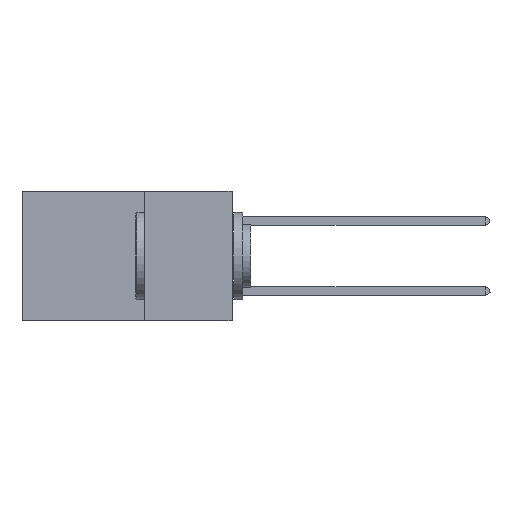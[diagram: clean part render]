
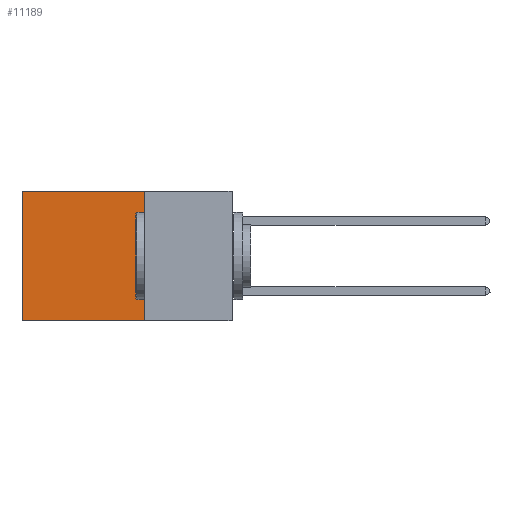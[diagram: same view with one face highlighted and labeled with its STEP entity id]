
A CAD part, left-side view. The second image highlights one B-rep face of the part: STEP entity #11189.
In plain terms, the highlighted planar face has unit normal (-1, 0, 0).
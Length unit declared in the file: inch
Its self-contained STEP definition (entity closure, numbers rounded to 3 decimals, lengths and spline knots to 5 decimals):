
#3844 = VECTOR ( 'NONE', #5964, 39.37008 ) ;
#5964 = DIRECTION ( 'NONE',  ( 0., 0., -1. ) ) ;
#8253 = EDGE_CURVE ( 'NONE', #15216, #16687, #18458, .T. ) ;
#8690 = CARTESIAN_POINT ( 'NONE',  ( 0.2875, 0.25, 0. ) ) ;
#9561 = EDGE_LOOP ( 'NONE', ( #16670, #21489, #13626, #18859 ) ) ;
#10514 = CARTESIAN_POINT ( 'NONE',  ( 0.2875, 0.25, 0. ) ) ;
#10618 = EDGE_CURVE ( 'NONE', #20994, #16687, #25148, .T. ) ;
#11189 = ADVANCED_FACE ( 'NONE', ( #21681 ), #18663, .F. ) ;
#11270 = VECTOR ( 'NONE', #27126, 39.37008 ) ;
#11901 = CARTESIAN_POINT ( 'NONE',  ( 0.2875, 0.25, 0. ) ) ;
#11990 = CARTESIAN_POINT ( 'NONE',  ( 0.2875, 0.25, -0.37 ) ) ;
#13626 = ORIENTED_EDGE ( 'NONE', *, *, #20654, .F. ) ;
#14032 = CARTESIAN_POINT ( 'NONE',  ( 0.2875, 0.6, 0. ) ) ;
#14743 = LINE ( 'NONE', #25379, #3844 ) ;
#15216 = VERTEX_POINT ( 'NONE', #17450 ) ;
#16177 = DIRECTION ( 'NONE',  ( 1., 0., 0. ) ) ;
#16329 = CARTESIAN_POINT ( 'NONE',  ( 0.2875, 0.6, -0.37 ) ) ;
#16400 = CARTESIAN_POINT ( 'NONE',  ( 0.2875, 0.6, 0. ) ) ;
#16670 = ORIENTED_EDGE ( 'NONE', *, *, #10618, .T. ) ;
#16687 = VERTEX_POINT ( 'NONE', #16329 ) ;
#17450 = CARTESIAN_POINT ( 'NONE',  ( 0.2875, 0.25, -0.37 ) ) ;
#18383 = AXIS2_PLACEMENT_3D ( 'NONE', #11901, #16177, #22835 ) ;
#18458 = LINE ( 'NONE', #11990, #11270 ) ;
#18600 = DIRECTION ( 'NONE',  ( 0., 0., -1. ) ) ;
#18604 = VERTEX_POINT ( 'NONE', #10514 ) ;
#18663 = PLANE ( 'NONE',  #18383 ) ;
#18859 = ORIENTED_EDGE ( 'NONE', *, *, #19291, .T. ) ;
#19291 = EDGE_CURVE ( 'NONE', #18604, #20994, #27669, .T. ) ;
#20654 = EDGE_CURVE ( 'NONE', #18604, #15216, #14743, .T. ) ;
#20994 = VERTEX_POINT ( 'NONE', #14032 ) ;
#21355 = VECTOR ( 'NONE', #18600, 39.37008 ) ;
#21489 = ORIENTED_EDGE ( 'NONE', *, *, #8253, .F. ) ;
#21681 = FACE_OUTER_BOUND ( 'NONE', #9561, .T. ) ;
#21850 = VECTOR ( 'NONE', #23705, 39.37008 ) ;
#22835 = DIRECTION ( 'NONE',  ( 0., 0., -1. ) ) ;
#23705 = DIRECTION ( 'NONE',  ( 0., 1., 0. ) ) ;
#25148 = LINE ( 'NONE', #16400, #21355 ) ;
#25379 = CARTESIAN_POINT ( 'NONE',  ( 0.2875, 0.25, 0. ) ) ;
#27126 = DIRECTION ( 'NONE',  ( 0., 1., 0. ) ) ;
#27669 = LINE ( 'NONE', #8690, #21850 ) ;
